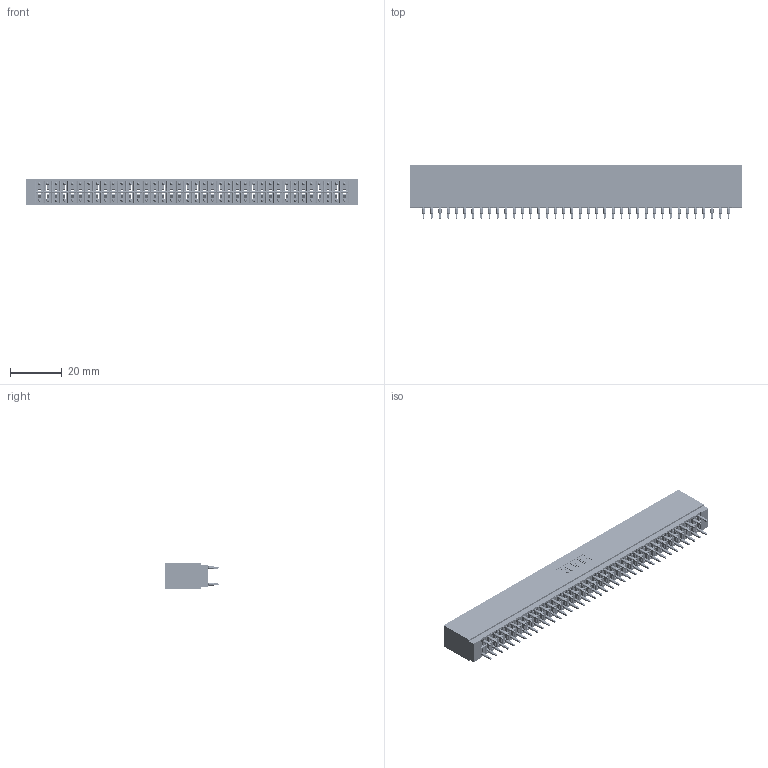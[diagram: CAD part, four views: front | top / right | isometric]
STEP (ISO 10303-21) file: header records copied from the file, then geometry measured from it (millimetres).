
FILE_DESCRIPTION (( 'STEP AP203' ), '1' );
FILE_NAME ('746-076-560-201.STEP', '2026-03-04T16:10:42', ( '' ), ( '' ), 'SwSTEP 2.0', 'SolidWorks 2023', '' );
FILE_SCHEMA (( 'CONFIG_CONTROL_DESIGN' ));
Length unit declared in the file: millimetre
Products named in the file (3): 746-292-001_560; 746 Part_.515 Slot Depth - 01; 746-076-560-201
Assembly tree (77 placements, depth 2):
  746-076-560-201
    746 Part_.515 Slot Depth - 01
    746-292-001_560  x76
Bounding box: 127.89 x 20.82 x 9.91 mm (x, y, z)
Volume: 13997.4 mm3; surface area: 23635.4 mm2
Topology: 77 solids, 77 shells, 7279 faces, 20251 edges, 12981 vertices
Faces by surface type: plane 3627, cylinder 1676, bspline 1520, torus 456
Entity records: 59392 total; most frequent: CARTESIAN_POINT 11839, ORIENTED_EDGE 10202, DIRECTION 8531, EDGE_CURVE 5101, VECTOR 4529, LINE 4529, VERTEX_POINT 3381, AXIS2_PLACEMENT_3D 2001
